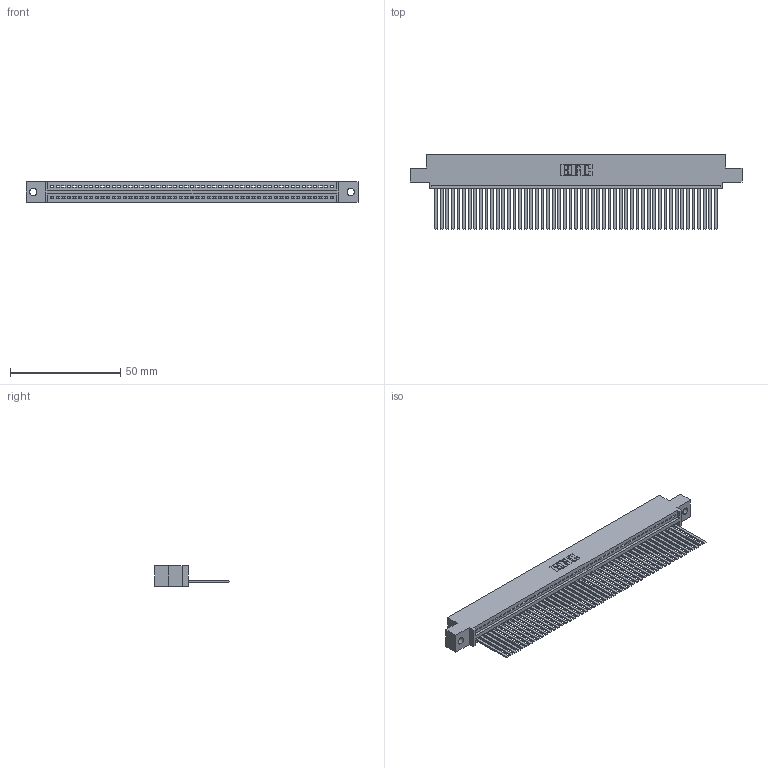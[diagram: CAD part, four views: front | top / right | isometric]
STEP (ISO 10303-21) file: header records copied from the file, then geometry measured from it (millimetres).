
FILE_DESCRIPTION (( 'STEP AP203' ), '1' );
FILE_NAME ('345-051-544-402.STEP', '2019-10-09T16:38:15', ( '' ), ( '' ), 'SwSTEP 2.0', 'SolidWorks 2016', '' );
FILE_SCHEMA (( 'CONFIG_CONTROL_DESIGN' ));
Length unit declared in the file: inch
Products named in the file (3): 345 Part_0.110 Offset - 0.128 Dia; 345-051-544-402; 345-292-001_345-293-144
Assembly tree (52 placements, depth 2):
  345-051-544-402
    345 Part_0.110 Offset - 0.128 Dia
    345-292-001_345-293-144  x51
Bounding box: 150.75 x 33.96 x 9.4 mm (x, y, z)
Volume: 14872.6 mm3; surface area: 21470.2 mm2
Topology: 52 solids, 52 shells, 2782 faces, 8411 edges, 5538 vertices
Faces by surface type: plane 1920, cylinder 862
Entity records: 37123 total; most frequent: CARTESIAN_POINT 6437, ORIENTED_EDGE 6422, DIRECTION 5605, EDGE_CURVE 3211, VECTOR 2879, LINE 2879, VERTEX_POINT 2138, AXIS2_PLACEMENT_3D 1363
